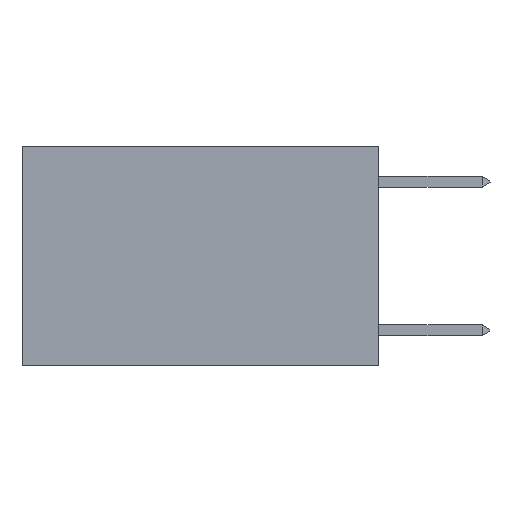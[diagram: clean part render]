
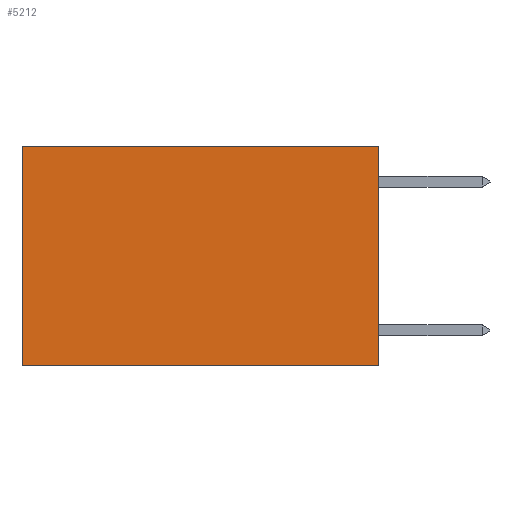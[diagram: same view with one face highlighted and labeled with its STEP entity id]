
A CAD part, left-side view. The second image highlights one B-rep face of the part: STEP entity #5212.
In plain terms, the highlighted planar face has unit normal (-1, 0, 0).
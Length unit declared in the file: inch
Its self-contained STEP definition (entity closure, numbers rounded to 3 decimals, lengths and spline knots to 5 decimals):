
#520 = LINE ( 'NONE', #6027, #13821 ) ;
#541 = EDGE_CURVE ( 'NONE', #10978, #1414, #4370, .T. ) ;
#745 = EDGE_CURVE ( 'NONE', #15772, #10978, #520, .T. ) ;
#1414 = VERTEX_POINT ( 'NONE', #2016 ) ;
#2016 = CARTESIAN_POINT ( 'NONE',  ( 0.2625, 0.6, -0.37 ) ) ;
#2141 = DIRECTION ( 'NONE',  ( 0., 1., 0. ) ) ;
#2516 = CARTESIAN_POINT ( 'NONE',  ( 0.2625, 0., 0. ) ) ;
#2626 = PLANE ( 'NONE',  #8571 ) ;
#3035 = DIRECTION ( 'NONE',  ( 0., 1., 0. ) ) ;
#3455 = VERTEX_POINT ( 'NONE', #3768 ) ;
#3508 = DIRECTION ( 'NONE',  ( 0., 0., -1. ) ) ;
#3768 = CARTESIAN_POINT ( 'NONE',  ( 0.2625, 0., -0.37 ) ) ;
#4039 = ORIENTED_EDGE ( 'NONE', *, *, #17470, .F. ) ;
#4370 = LINE ( 'NONE', #14208, #8246 ) ;
#5212 = ADVANCED_FACE ( 'NONE', ( #6623 ), #2626, .F. ) ;
#5535 = ORIENTED_EDGE ( 'NONE', *, *, #541, .T. ) ;
#6027 = CARTESIAN_POINT ( 'NONE',  ( 0.2625, 0., 0. ) ) ;
#6623 = FACE_OUTER_BOUND ( 'NONE', #14591, .T. ) ;
#6713 = DIRECTION ( 'NONE',  ( 1., 0., 0. ) ) ;
#8246 = VECTOR ( 'NONE', #11464, 39.37008 ) ;
#8256 = DIRECTION ( 'NONE',  ( 0., 0., -1. ) ) ;
#8571 = AXIS2_PLACEMENT_3D ( 'NONE', #9510, #6713, #8256 ) ;
#9510 = CARTESIAN_POINT ( 'NONE',  ( 0.2625, 0., 0. ) ) ;
#9664 = VECTOR ( 'NONE', #3508, 39.37008 ) ;
#10978 = VERTEX_POINT ( 'NONE', #14456 ) ;
#11159 = VECTOR ( 'NONE', #2141, 39.37008 ) ;
#11376 = ORIENTED_EDGE ( 'NONE', *, *, #745, .T. ) ;
#11464 = DIRECTION ( 'NONE',  ( 0., 0., -1. ) ) ;
#11710 = ORIENTED_EDGE ( 'NONE', *, *, #15623, .F. ) ;
#12410 = CARTESIAN_POINT ( 'NONE',  ( 0.2625, 0., 0. ) ) ;
#13821 = VECTOR ( 'NONE', #3035, 39.37008 ) ;
#14208 = CARTESIAN_POINT ( 'NONE',  ( 0.2625, 0.6, 0. ) ) ;
#14456 = CARTESIAN_POINT ( 'NONE',  ( 0.2625, 0.6, 0. ) ) ;
#14591 = EDGE_LOOP ( 'NONE', ( #5535, #4039, #11710, #11376 ) ) ;
#14615 = LINE ( 'NONE', #2516, #9664 ) ;
#15623 = EDGE_CURVE ( 'NONE', #15772, #3455, #14615, .T. ) ;
#15772 = VERTEX_POINT ( 'NONE', #12410 ) ;
#16053 = LINE ( 'NONE', #17597, #11159 ) ;
#17470 = EDGE_CURVE ( 'NONE', #3455, #1414, #16053, .T. ) ;
#17597 = CARTESIAN_POINT ( 'NONE',  ( 0.2625, 0., -0.37 ) ) ;
